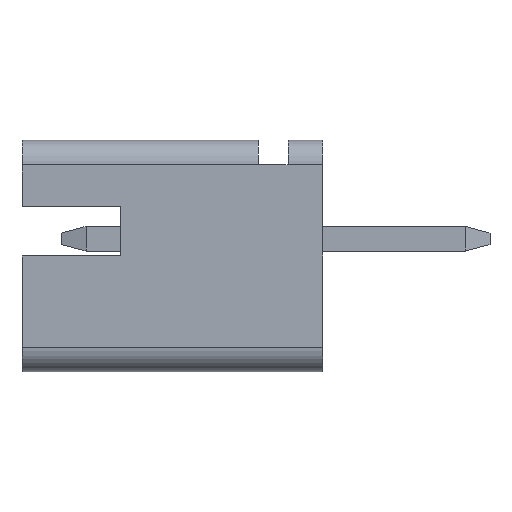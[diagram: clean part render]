
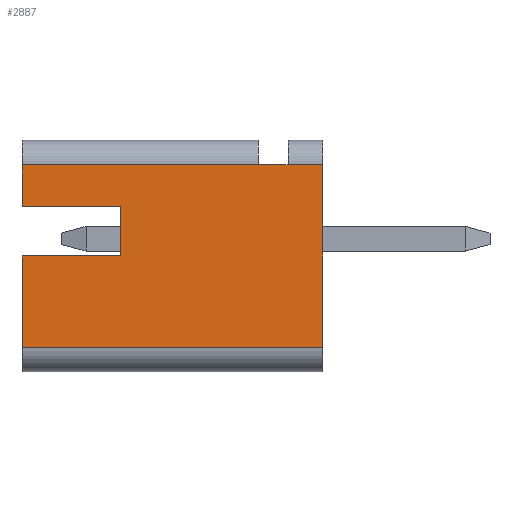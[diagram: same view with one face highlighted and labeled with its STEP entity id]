
A CAD part, left-side view. The second image highlights one B-rep face of the part: STEP entity #2887.
In plain terms, the highlighted planar face has unit normal (-1, 0, 0).
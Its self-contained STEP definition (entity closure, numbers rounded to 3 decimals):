
#6 = DIRECTION ( 'NONE',  ( 0., 0., 1. ) ) ;
#50 = CARTESIAN_POINT ( 'NONE',  ( -2., 6.1, -2.2 ) ) ;
#63 = LINE ( 'NONE', #1073, #593 ) ;
#123 = DIRECTION ( 'NONE',  ( 0., 0., 1. ) ) ;
#141 = LINE ( 'NONE', #1588, #194 ) ;
#189 = CARTESIAN_POINT ( 'NONE',  ( -2., 6.1, 1.5 ) ) ;
#194 = VECTOR ( 'NONE', #2838, 1000. ) ;
#236 = CARTESIAN_POINT ( 'NONE',  ( -2., 0., 1.5 ) ) ;
#262 = LINE ( 'NONE', #2368, #2842 ) ;
#274 = VECTOR ( 'NONE', #2623, 1000. ) ;
#325 = ORIENTED_EDGE ( 'NONE', *, *, #2238, .F. ) ;
#338 = DIRECTION ( 'NONE',  ( 0., 0., 1. ) ) ;
#411 = EDGE_LOOP ( 'NONE', ( #727, #956, #325, #3129, #1564, #770, #2569, #2612, #1088, #2220 ) ) ;
#430 = VECTOR ( 'NONE', #2834, 1000. ) ;
#471 = CARTESIAN_POINT ( 'NONE',  ( -2., 1.3, 1.5 ) ) ;
#551 = CARTESIAN_POINT ( 'NONE',  ( -2., 0.7, 1.5 ) ) ;
#573 = CARTESIAN_POINT ( 'NONE',  ( -2., 0., 1.5 ) ) ;
#593 = VECTOR ( 'NONE', #338, 1000. ) ;
#598 = EDGE_CURVE ( 'NONE', #2896, #944, #1466, .T. ) ;
#610 = VERTEX_POINT ( 'NONE', #50 ) ;
#624 = LINE ( 'NONE', #2826, #1218 ) ;
#727 = ORIENTED_EDGE ( 'NONE', *, *, #1659, .F. ) ;
#770 = ORIENTED_EDGE ( 'NONE', *, *, #2635, .T. ) ;
#787 = VERTEX_POINT ( 'NONE', #573 ) ;
#827 = VECTOR ( 'NONE', #2204, 1000. ) ;
#896 = CARTESIAN_POINT ( 'NONE',  ( -2., 1.3, 1.5 ) ) ;
#917 = EDGE_CURVE ( 'NONE', #2955, #1340, #63, .T. ) ;
#944 = VERTEX_POINT ( 'NONE', #551 ) ;
#956 = ORIENTED_EDGE ( 'NONE', *, *, #1806, .T. ) ;
#968 = CARTESIAN_POINT ( 'NONE',  ( -2., 0., -2.2 ) ) ;
#981 = CARTESIAN_POINT ( 'NONE',  ( -2., 6.1, -0.35 ) ) ;
#990 = EDGE_CURVE ( 'NONE', #1340, #1081, #141, .T. ) ;
#1073 = CARTESIAN_POINT ( 'NONE',  ( -2., 4.1, 0.65 ) ) ;
#1081 = VERTEX_POINT ( 'NONE', #2545 ) ;
#1088 = ORIENTED_EDGE ( 'NONE', *, *, #917, .F. ) ;
#1142 = VECTOR ( 'NONE', #1463, 1000. ) ;
#1179 = VECTOR ( 'NONE', #123, 1000. ) ;
#1218 = VECTOR ( 'NONE', #2763, 1000. ) ;
#1276 = CARTESIAN_POINT ( 'NONE',  ( -2., 0., -2.2 ) ) ;
#1340 = VERTEX_POINT ( 'NONE', #2272 ) ;
#1343 = CARTESIAN_POINT ( 'NONE',  ( -2., 0., 2. ) ) ;
#1347 = FACE_OUTER_BOUND ( 'NONE', #411, .T. ) ;
#1380 = DIRECTION ( 'NONE',  ( 1., 0., 0. ) ) ;
#1401 = VERTEX_POINT ( 'NONE', #1276 ) ;
#1405 = LINE ( 'NONE', #236, #274 ) ;
#1463 = DIRECTION ( 'NONE',  ( 0., -1., 0. ) ) ;
#1466 = LINE ( 'NONE', #471, #827 ) ;
#1564 = ORIENTED_EDGE ( 'NONE', *, *, #598, .F. ) ;
#1586 = LINE ( 'NONE', #1343, #430 ) ;
#1588 = CARTESIAN_POINT ( 'NONE',  ( -2., 6.1, 0.65 ) ) ;
#1609 = CARTESIAN_POINT ( 'NONE',  ( -2., 6.1, -0.35 ) ) ;
#1642 = DIRECTION ( 'NONE',  ( 0., 0., -1. ) ) ;
#1659 = EDGE_CURVE ( 'NONE', #610, #2850, #262, .T. ) ;
#1674 = DIRECTION ( 'NONE',  ( 0., -1., 0. ) ) ;
#1806 = EDGE_CURVE ( 'NONE', #610, #1401, #2409, .T. ) ;
#1823 = CARTESIAN_POINT ( 'NONE',  ( -2., 4.1, -0.35 ) ) ;
#1873 = PLANE ( 'NONE',  #2228 ) ;
#1969 = EDGE_CURVE ( 'NONE', #2850, #2955, #2616, .T. ) ;
#2109 = CARTESIAN_POINT ( 'NONE',  ( -2., 0., 0. ) ) ;
#2169 = EDGE_CURVE ( 'NONE', #1081, #3036, #2289, .T. ) ;
#2204 = DIRECTION ( 'NONE',  ( 0., -1., 0. ) ) ;
#2220 = ORIENTED_EDGE ( 'NONE', *, *, #1969, .F. ) ;
#2228 = AXIS2_PLACEMENT_3D ( 'NONE', #2109, #1380, #1642 ) ;
#2238 = EDGE_CURVE ( 'NONE', #787, #1401, #1586, .T. ) ;
#2272 = CARTESIAN_POINT ( 'NONE',  ( -2., 4.1, 0.65 ) ) ;
#2289 = LINE ( 'NONE', #2782, #1179 ) ;
#2351 = VECTOR ( 'NONE', #1674, 1000. ) ;
#2368 = CARTESIAN_POINT ( 'NONE',  ( -2., 6.1, -0.35 ) ) ;
#2377 = EDGE_CURVE ( 'NONE', #787, #944, #1405, .T. ) ;
#2409 = LINE ( 'NONE', #968, #2351 ) ;
#2545 = CARTESIAN_POINT ( 'NONE',  ( -2., 6.1, 0.65 ) ) ;
#2569 = ORIENTED_EDGE ( 'NONE', *, *, #2169, .F. ) ;
#2612 = ORIENTED_EDGE ( 'NONE', *, *, #990, .F. ) ;
#2616 = LINE ( 'NONE', #981, #1142 ) ;
#2623 = DIRECTION ( 'NONE',  ( 0., 1., 0. ) ) ;
#2635 = EDGE_CURVE ( 'NONE', #2896, #3036, #624, .T. ) ;
#2763 = DIRECTION ( 'NONE',  ( 0., 1., 0. ) ) ;
#2782 = CARTESIAN_POINT ( 'NONE',  ( -2., 6.1, 2. ) ) ;
#2826 = CARTESIAN_POINT ( 'NONE',  ( -2., 0., 1.5 ) ) ;
#2834 = DIRECTION ( 'NONE',  ( 0., 0., -1. ) ) ;
#2838 = DIRECTION ( 'NONE',  ( 0., 1., 0. ) ) ;
#2842 = VECTOR ( 'NONE', #6, 1000. ) ;
#2850 = VERTEX_POINT ( 'NONE', #1609 ) ;
#2887 = ADVANCED_FACE ( 'NONE', ( #1347 ), #1873, .F. ) ;
#2896 = VERTEX_POINT ( 'NONE', #896 ) ;
#2955 = VERTEX_POINT ( 'NONE', #1823 ) ;
#3036 = VERTEX_POINT ( 'NONE', #189 ) ;
#3129 = ORIENTED_EDGE ( 'NONE', *, *, #2377, .T. ) ;
